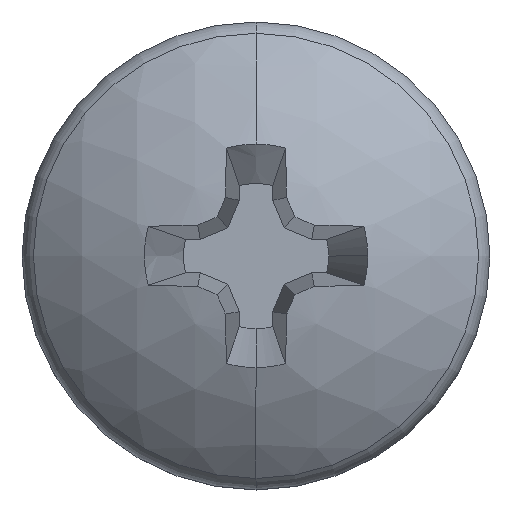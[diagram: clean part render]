
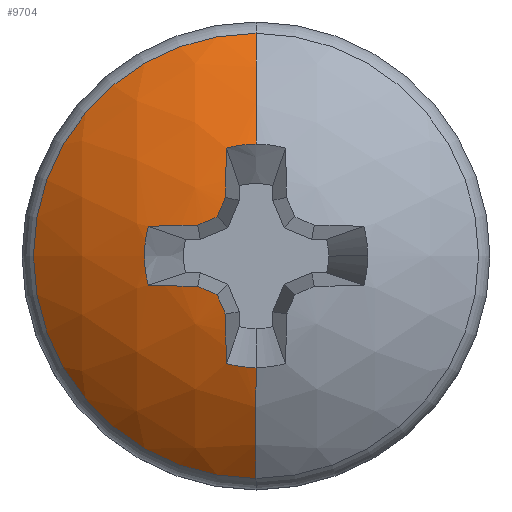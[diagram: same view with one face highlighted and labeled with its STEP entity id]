
A CAD part, top view. The second image highlights one B-rep face of the part: STEP entity #9704.
In plain terms, the highlighted spherical face has radius 4.225 mm.
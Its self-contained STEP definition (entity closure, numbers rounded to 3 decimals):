
#19 = CARTESIAN_POINT ( 'NONE',  ( -0.749, 0.393, 32.415 ) ) ;
#121 = CARTESIAN_POINT ( 'NONE',  ( 0., 1.433, 32.25 ) ) ;
#125 = AXIS2_PLACEMENT_3D ( 'NONE', #7348, #16330, #8655 ) ;
#445 = DIRECTION ( 'NONE',  ( 1., 0., 0. ) ) ;
#481 = CIRCLE ( 'NONE', #3242, 4.225 ) ;
#653 = AXIS2_PLACEMENT_3D ( 'NONE', #14583, #6888, #15880 ) ;
#847 = CARTESIAN_POINT ( 'NONE',  ( -0.03, 0., 28.272 ) ) ;
#898 = CARTESIAN_POINT ( 'NONE',  ( -0.499, 0.499, 32.441 ) ) ;
#980 = CIRCLE ( 'NONE', #15344, 4.225 ) ;
#1036 = EDGE_CURVE ( 'NONE', #2792, #3854, #980, .T. ) ;
#1158 = CARTESIAN_POINT ( 'NONE',  ( -0.378, -1.382, 32.25 ) ) ;
#1196 = ORIENTED_EDGE ( 'NONE', *, *, #16540, .F. ) ;
#1241 = ORIENTED_EDGE ( 'NONE', *, *, #1259, .F. ) ;
#1245 = DIRECTION ( 'NONE',  ( -0.383, 0.924, 0. ) ) ;
#1259 = EDGE_CURVE ( 'NONE', #11306, #11711, #5017, .T. ) ;
#1447 = AXIS2_PLACEMENT_3D ( 'NONE', #4852, #13821, #6130 ) ;
#1953 = CARTESIAN_POINT ( 'NONE',  ( 0., 0., 32.25 ) ) ;
#2082 = EDGE_CURVE ( 'NONE', #11711, #2193, #14905, .T. ) ;
#2115 = DIRECTION ( 'NONE',  ( 0.087, 0., -0.996 ) ) ;
#2193 = VERTEX_POINT ( 'NONE', #5343 ) ;
#2356 = ORIENTED_EDGE ( 'NONE', *, *, #4385, .T. ) ;
#2730 = EDGE_CURVE ( 'NONE', #3854, #5266, #9267, .T. ) ;
#2752 = DIRECTION ( 'NONE',  ( 0., 0., 1. ) ) ;
#2792 = VERTEX_POINT ( 'NONE', #5253 ) ;
#3213 = VERTEX_POINT ( 'NONE', #14006 ) ;
#3242 = AXIS2_PLACEMENT_3D ( 'NONE', #847, #9868, #2115 ) ;
#3252 = DIRECTION ( 'NONE',  ( 0., 1., 0. ) ) ;
#3486 = AXIS2_PLACEMENT_3D ( 'NONE', #16632, #8981, #1245 ) ;
#3729 = CARTESIAN_POINT ( 'NONE',  ( 0., -2.854, 31.39 ) ) ;
#3776 = CARTESIAN_POINT ( 'NONE',  ( 0., 0., 32.25 ) ) ;
#3854 = VERTEX_POINT ( 'NONE', #121 ) ;
#4014 = CARTESIAN_POINT ( 'NONE',  ( -0.393, 0.749, 32.415 ) ) ;
#4101 = DIRECTION ( 'NONE',  ( 0.381, -0.92, 0.087 ) ) ;
#4169 = EDGE_CURVE ( 'NONE', #9902, #3213, #5792, .T. ) ;
#4245 = VERTEX_POINT ( 'NONE', #1158 ) ;
#4385 = EDGE_CURVE ( 'NONE', #2792, #6261, #10248, .T. ) ;
#4647 = ORIENTED_EDGE ( 'NONE', *, *, #15904, .T. ) ;
#4852 = CARTESIAN_POINT ( 'NONE',  ( -0.03, 0., 28.272 ) ) ;
#4878 = VERTEX_POINT ( 'NONE', #898 ) ;
#4898 = ORIENTED_EDGE ( 'NONE', *, *, #2082, .F. ) ;
#4971 = AXIS2_PLACEMENT_3D ( 'NONE', #10512, #2752, #11785 ) ;
#5017 = CIRCLE ( 'NONE', #15860, 4.215 ) ;
#5070 = DIRECTION ( 'NONE',  ( -0.924, 0.383, 0. ) ) ;
#5075 = DIRECTION ( 'NONE',  ( 0.381, 0.92, 0.087 ) ) ;
#5093 = DIRECTION ( 'NONE',  ( -1., 0., 0. ) ) ;
#5095 = DIRECTION ( 'NONE',  ( -1., 0., 0. ) ) ;
#5187 = ORIENTED_EDGE ( 'NONE', *, *, #1036, .F. ) ;
#5253 = CARTESIAN_POINT ( 'NONE',  ( 0., 2.854, 31.39 ) ) ;
#5266 = VERTEX_POINT ( 'NONE', #13166 ) ;
#5291 = DIRECTION ( 'NONE',  ( 0., 0.996, 0.087 ) ) ;
#5336 = AXIS2_PLACEMENT_3D ( 'NONE', #12784, #5095, #14085 ) ;
#5343 = CARTESIAN_POINT ( 'NONE',  ( -0.393, -0.749, 32.415 ) ) ;
#5464 = AXIS2_PLACEMENT_3D ( 'NONE', #12990, #5291, #14281 ) ;
#5792 = CIRCLE ( 'NONE', #125, 4.225 ) ;
#5829 = ORIENTED_EDGE ( 'NONE', *, *, #11924, .F. ) ;
#5879 = EDGE_CURVE ( 'NONE', #3213, #6274, #9391, .T. ) ;
#6130 = DIRECTION ( 'NONE',  ( 0.087, 0., -0.996 ) ) ;
#6258 = DIRECTION ( 'NONE',  ( 0.92, -0.381, 0.087 ) ) ;
#6261 = VERTEX_POINT ( 'NONE', #3729 ) ;
#6274 = VERTEX_POINT ( 'NONE', #15445 ) ;
#6456 = VERTEX_POINT ( 'NONE', #12153 ) ;
#6521 = CIRCLE ( 'NONE', #8712, 4.215 ) ;
#6814 = ORIENTED_EDGE ( 'NONE', *, *, #9657, .F. ) ;
#6888 = DIRECTION ( 'NONE',  ( 0., 0., 1. ) ) ;
#7348 = CARTESIAN_POINT ( 'NONE',  ( 0., 0.03, 28.272 ) ) ;
#7644 = CIRCLE ( 'NONE', #5336, 4.225 ) ;
#8158 = EDGE_CURVE ( 'NONE', #2193, #4245, #11611, .T. ) ;
#8162 = CARTESIAN_POINT ( 'NONE',  ( 0., 0., 28.275 ) ) ;
#8253 = AXIS2_PLACEMENT_3D ( 'NONE', #3776, #12783, #5093 ) ;
#8459 = CARTESIAN_POINT ( 'NONE',  ( -0.499, -0.499, 32.441 ) ) ;
#8655 = DIRECTION ( 'NONE',  ( 0., -0.087, -0.996 ) ) ;
#8712 = AXIS2_PLACEMENT_3D ( 'NONE', #11812, #4101, #13105 ) ;
#8981 = DIRECTION ( 'NONE',  ( 0.92, 0.381, 0.087 ) ) ;
#9267 = CIRCLE ( 'NONE', #8253, 1.433 ) ;
#9320 = AXIS2_PLACEMENT_3D ( 'NONE', #16362, #12441, #13850 ) ;
#9391 = CIRCLE ( 'NONE', #653, 1.433 ) ;
#9447 = CARTESIAN_POINT ( 'NONE',  ( -0.109, -0.263, 28.25 ) ) ;
#9452 = DIRECTION ( 'NONE',  ( 0., 0., -1. ) ) ;
#9657 = EDGE_CURVE ( 'NONE', #5266, #10319, #481, .T. ) ;
#9704 = ADVANCED_FACE ( 'NONE', ( #12974 ), #16381, .T. ) ;
#9868 = DIRECTION ( 'NONE',  ( 0.996, 0., 0.087 ) ) ;
#9875 = ORIENTED_EDGE ( 'NONE', *, *, #14196, .F. ) ;
#9902 = VERTEX_POINT ( 'NONE', #19 ) ;
#9943 = CARTESIAN_POINT ( 'NONE',  ( -0.749, -0.393, 32.415 ) ) ;
#10248 = CIRCLE ( 'NONE', #4971, 2.854 ) ;
#10319 = VERTEX_POINT ( 'NONE', #4014 ) ;
#10512 = CARTESIAN_POINT ( 'NONE',  ( 0., 0., 31.39 ) ) ;
#10715 = AXIS2_PLACEMENT_3D ( 'NONE', #13950, #6258, #15245 ) ;
#10982 = DIRECTION ( 'NONE',  ( 0., 0., 1. ) ) ;
#11306 = VERTEX_POINT ( 'NONE', #9943 ) ;
#11611 = CIRCLE ( 'NONE', #1447, 4.225 ) ;
#11686 = CIRCLE ( 'NONE', #10715, 4.215 ) ;
#11711 = VERTEX_POINT ( 'NONE', #8459 ) ;
#11785 = DIRECTION ( 'NONE',  ( 0., -1., 0. ) ) ;
#11812 = CARTESIAN_POINT ( 'NONE',  ( -0.109, 0.263, 28.25 ) ) ;
#11851 = ORIENTED_EDGE ( 'NONE', *, *, #2730, .F. ) ;
#11924 = EDGE_CURVE ( 'NONE', #6274, #11306, #12124, .T. ) ;
#12124 = CIRCLE ( 'NONE', #5464, 4.225 ) ;
#12153 = CARTESIAN_POINT ( 'NONE',  ( 0., -1.433, 32.25 ) ) ;
#12441 = DIRECTION ( 'NONE',  ( -1., 0., 0. ) ) ;
#12783 = DIRECTION ( 'NONE',  ( 0., 0., 1. ) ) ;
#12784 = CARTESIAN_POINT ( 'NONE',  ( 0., 0., 28.275 ) ) ;
#12974 = FACE_OUTER_BOUND ( 'NONE', #15284, .T. ) ;
#12990 = CARTESIAN_POINT ( 'NONE',  ( 0., -0.03, 28.272 ) ) ;
#13105 = DIRECTION ( 'NONE',  ( 0.924, 0.383, 0. ) ) ;
#13166 = CARTESIAN_POINT ( 'NONE',  ( -0.378, 1.382, 32.25 ) ) ;
#13483 = CIRCLE ( 'NONE', #14865, 1.433 ) ;
#13821 = DIRECTION ( 'NONE',  ( 0.996, 0., 0.087 ) ) ;
#13850 = DIRECTION ( 'NONE',  ( 0., 1., 0. ) ) ;
#13950 = CARTESIAN_POINT ( 'NONE',  ( -0.263, 0.109, 28.25 ) ) ;
#14006 = CARTESIAN_POINT ( 'NONE',  ( -1.382, 0.378, 32.25 ) ) ;
#14085 = DIRECTION ( 'NONE',  ( 0., -1., 0. ) ) ;
#14196 = EDGE_CURVE ( 'NONE', #4245, #6456, #13483, .T. ) ;
#14281 = DIRECTION ( 'NONE',  ( 0., -0.087, 0.996 ) ) ;
#14583 = CARTESIAN_POINT ( 'NONE',  ( 0., 0., 32.25 ) ) ;
#14821 = EDGE_CURVE ( 'NONE', #10319, #4878, #11686, .T. ) ;
#14865 = AXIS2_PLACEMENT_3D ( 'NONE', #1953, #10982, #3252 ) ;
#14905 = CIRCLE ( 'NONE', #3486, 4.215 ) ;
#15245 = DIRECTION ( 'NONE',  ( 0.383, 0.924, 0. ) ) ;
#15284 = EDGE_LOOP ( 'NONE', ( #2356, #4647, #9875, #16341, #4898, #1241, #5829, #16145, #16234, #1196, #15521, #6814, #11851, #5187 ) ) ;
#15344 = AXIS2_PLACEMENT_3D ( 'NONE', #8162, #445, #9452 ) ;
#15445 = CARTESIAN_POINT ( 'NONE',  ( -1.382, -0.378, 32.25 ) ) ;
#15521 = ORIENTED_EDGE ( 'NONE', *, *, #14821, .F. ) ;
#15860 = AXIS2_PLACEMENT_3D ( 'NONE', #9447, #5075, #5070 ) ;
#15880 = DIRECTION ( 'NONE',  ( -1., 0., 0. ) ) ;
#15904 = EDGE_CURVE ( 'NONE', #6261, #6456, #7644, .T. ) ;
#16145 = ORIENTED_EDGE ( 'NONE', *, *, #5879, .F. ) ;
#16234 = ORIENTED_EDGE ( 'NONE', *, *, #4169, .F. ) ;
#16330 = DIRECTION ( 'NONE',  ( 0., -0.996, 0.087 ) ) ;
#16341 = ORIENTED_EDGE ( 'NONE', *, *, #8158, .F. ) ;
#16362 = CARTESIAN_POINT ( 'NONE',  ( 0., 0., 28.275 ) ) ;
#16381 = SPHERICAL_SURFACE ( 'NONE', #9320, 4.225 ) ;
#16540 = EDGE_CURVE ( 'NONE', #4878, #9902, #6521, .T. ) ;
#16632 = CARTESIAN_POINT ( 'NONE',  ( -0.263, -0.109, 28.25 ) ) ;
